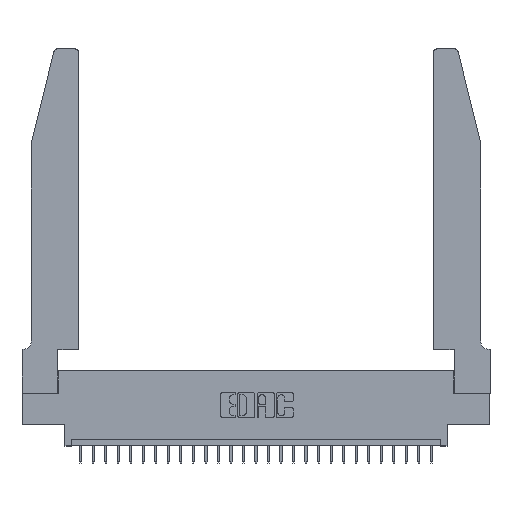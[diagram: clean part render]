
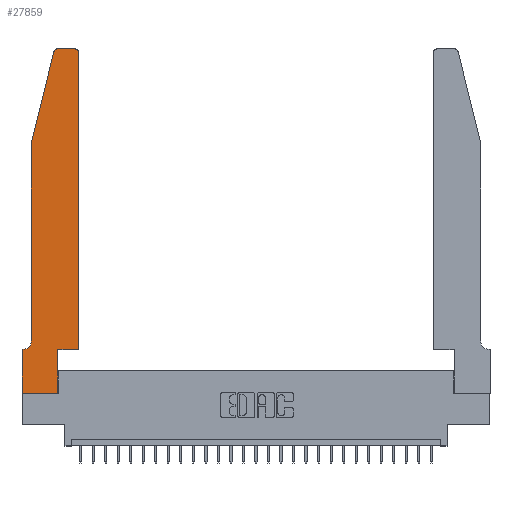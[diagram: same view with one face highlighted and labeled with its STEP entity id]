
A CAD part, top view. The second image highlights one B-rep face of the part: STEP entity #27859.
In plain terms, the highlighted planar face has unit normal (0, 0, 1).
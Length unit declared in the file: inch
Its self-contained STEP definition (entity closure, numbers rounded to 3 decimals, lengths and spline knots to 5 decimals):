
#361 = CARTESIAN_POINT ( 'NONE',  ( 0.4505, 0.35, 0.37 ) ) ;
#369 = AXIS2_PLACEMENT_3D ( 'NONE', #16245, #648, #2953 ) ;
#456 = LINE ( 'NONE', #11005, #26576 ) ;
#542 = LINE ( 'NONE', #18166, #25322 ) ;
#648 = DIRECTION ( 'NONE',  ( 0., 0., -1. ) ) ;
#783 = DIRECTION ( 'NONE',  ( 1., 0., 0. ) ) ;
#1442 = VECTOR ( 'NONE', #6772, 39.37008 ) ;
#1499 = VECTOR ( 'NONE', #19716, 39.37008 ) ;
#1533 = EDGE_CURVE ( 'NONE', #22584, #27762, #24701, .T. ) ;
#1870 = VERTEX_POINT ( 'NONE', #19478 ) ;
#1939 = PLANE ( 'NONE',  #6415 ) ;
#2054 = VERTEX_POINT ( 'NONE', #26553 ) ;
#2544 = DIRECTION ( 'NONE',  ( -0.239, -0.971, 0. ) ) ;
#2953 = DIRECTION ( 'NONE',  ( -1., 0., 0. ) ) ;
#3086 = ORIENTED_EDGE ( 'NONE', *, *, #11861, .T. ) ;
#3367 = CARTESIAN_POINT ( 'NONE',  ( 0.284, 2.72, 0.37 ) ) ;
#3793 = EDGE_CURVE ( 'NONE', #7528, #2054, #24364, .T. ) ;
#4366 = ORIENTED_EDGE ( 'NONE', *, *, #24032, .T. ) ;
#4650 = CARTESIAN_POINT ( 'NONE',  ( 0., 0., 0.37 ) ) ;
#4769 = VECTOR ( 'NONE', #24494, 39.37008 ) ;
#5351 = VECTOR ( 'NONE', #783, 39.37008 ) ;
#5953 = ORIENTED_EDGE ( 'NONE', *, *, #17704, .T. ) ;
#6149 = ORIENTED_EDGE ( 'NONE', *, *, #26749, .T. ) ;
#6403 = CARTESIAN_POINT ( 'NONE',  ( 0., 0.35, 0.37 ) ) ;
#6415 = AXIS2_PLACEMENT_3D ( 'NONE', #6403, #8720, #15228 ) ;
#6772 = DIRECTION ( 'NONE',  ( -1., 0., 0. ) ) ;
#7038 = CARTESIAN_POINT ( 'NONE',  ( 0., 0., 0.37 ) ) ;
#7094 = DIRECTION ( 'NONE',  ( 1., 0., 0. ) ) ;
#7528 = VERTEX_POINT ( 'NONE', #22080 ) ;
#7736 = VERTEX_POINT ( 'NONE', #20895 ) ;
#7796 = VERTEX_POINT ( 'NONE', #15268 ) ;
#8121 = ORIENTED_EDGE ( 'NONE', *, *, #8553, .T. ) ;
#8229 = CIRCLE ( 'NONE', #20662, 0.03 ) ;
#8553 = EDGE_CURVE ( 'NONE', #8841, #7736, #11332, .T. ) ;
#8720 = DIRECTION ( 'NONE',  ( 0., 0., 1. ) ) ;
#8841 = VERTEX_POINT ( 'NONE', #23744 ) ;
#9435 = VECTOR ( 'NONE', #7094, 39.37008 ) ;
#9494 = VECTOR ( 'NONE', #2544, 39.37008 ) ;
#9614 = LINE ( 'NONE', #13514, #9494 ) ;
#10601 = FACE_OUTER_BOUND ( 'NONE', #12995, .T. ) ;
#10947 = EDGE_CURVE ( 'NONE', #2054, #22584, #14672, .T. ) ;
#11005 = CARTESIAN_POINT ( 'NONE',  ( 0.2605, 2.75, 0.37 ) ) ;
#11064 = CARTESIAN_POINT ( 'NONE',  ( 0.0755, 2., 0.37 ) ) ;
#11247 = AXIS2_PLACEMENT_3D ( 'NONE', #15539, #28255, #28542 ) ;
#11257 = CARTESIAN_POINT ( 'NONE',  ( 0.0755, 0.35, 0.37 ) ) ;
#11332 = LINE ( 'NONE', #361, #5351 ) ;
#11582 = CARTESIAN_POINT ( 'NONE',  ( 0., 0., 0.37 ) ) ;
#11703 = CIRCLE ( 'NONE', #11247, 0.03 ) ;
#11861 = EDGE_CURVE ( 'NONE', #7736, #20098, #542, .T. ) ;
#12822 = VERTEX_POINT ( 'NONE', #11582 ) ;
#12995 = EDGE_LOOP ( 'NONE', ( #4366, #6149, #25354, #23075, #25969, #13064, #5953, #27306, #22195, #8121, #3086, #13668 ) ) ;
#13064 = ORIENTED_EDGE ( 'NONE', *, *, #1533, .T. ) ;
#13514 = CARTESIAN_POINT ( 'NONE',  ( 0.0755, 2., 0.37 ) ) ;
#13668 = ORIENTED_EDGE ( 'NONE', *, *, #19941, .T. ) ;
#13795 = CARTESIAN_POINT ( 'NONE',  ( 0.0055, 0.35, 0.37 ) ) ;
#14672 = CIRCLE ( 'NONE', #369, 0.07 ) ;
#15228 = DIRECTION ( 'NONE',  ( 1., 0., 0. ) ) ;
#15268 = CARTESIAN_POINT ( 'NONE',  ( 0.25487, 2.72718, 0.37 ) ) ;
#15539 = CARTESIAN_POINT ( 'NONE',  ( 0.4205, 2.72, 0.37 ) ) ;
#15995 = DIRECTION ( 'NONE',  ( 0., 1., 0. ) ) ;
#16245 = CARTESIAN_POINT ( 'NONE',  ( 0.0055, 0.42, 0.37 ) ) ;
#16806 = DIRECTION ( 'NONE',  ( 1., 0., 0. ) ) ;
#17084 = DIRECTION ( 'NONE',  ( 0., 0., 1. ) ) ;
#17645 = DIRECTION ( 'NONE',  ( -1., 0., 0. ) ) ;
#17704 = EDGE_CURVE ( 'NONE', #27762, #12822, #20059, .T. ) ;
#18166 = CARTESIAN_POINT ( 'NONE',  ( 0.4505, 0.35, 0.37 ) ) ;
#18259 = EDGE_CURVE ( 'NONE', #25081, #8841, #24197, .T. ) ;
#19478 = CARTESIAN_POINT ( 'NONE',  ( 0.4205, 2.75, 0.37 ) ) ;
#19561 = CARTESIAN_POINT ( 'NONE',  ( 0., 0.35, 0.37 ) ) ;
#19716 = DIRECTION ( 'NONE',  ( 0., 1., 0. ) ) ;
#19941 = EDGE_CURVE ( 'NONE', #20098, #1870, #11703, .T. ) ;
#20059 = LINE ( 'NONE', #7038, #24100 ) ;
#20098 = VERTEX_POINT ( 'NONE', #24920 ) ;
#20490 = EDGE_CURVE ( 'NONE', #12822, #25081, #26753, .T. ) ;
#20662 = AXIS2_PLACEMENT_3D ( 'NONE', #3367, #17084, #16806 ) ;
#20782 = CARTESIAN_POINT ( 'NONE',  ( 0.2865, 0., 0.37 ) ) ;
#20895 = CARTESIAN_POINT ( 'NONE',  ( 0.4505, 0.35, 0.37 ) ) ;
#21125 = VERTEX_POINT ( 'NONE', #23063 ) ;
#22080 = CARTESIAN_POINT ( 'NONE',  ( 0.0755, 2., 0.37 ) ) ;
#22195 = ORIENTED_EDGE ( 'NONE', *, *, #18259, .T. ) ;
#22584 = VERTEX_POINT ( 'NONE', #13795 ) ;
#23063 = CARTESIAN_POINT ( 'NONE',  ( 0.284, 2.75, 0.37 ) ) ;
#23075 = ORIENTED_EDGE ( 'NONE', *, *, #3793, .T. ) ;
#23744 = CARTESIAN_POINT ( 'NONE',  ( 0.2865, 0.35, 0.37 ) ) ;
#23829 = EDGE_CURVE ( 'NONE', #7796, #7528, #9614, .T. ) ;
#24032 = EDGE_CURVE ( 'NONE', #1870, #21125, #456, .T. ) ;
#24100 = VECTOR ( 'NONE', #26988, 39.37008 ) ;
#24197 = LINE ( 'NONE', #28239, #1499 ) ;
#24364 = LINE ( 'NONE', #11064, #4769 ) ;
#24494 = DIRECTION ( 'NONE',  ( 0., -1., 0. ) ) ;
#24701 = LINE ( 'NONE', #11257, #1442 ) ;
#24920 = CARTESIAN_POINT ( 'NONE',  ( 0.4505, 2.72, 0.37 ) ) ;
#25081 = VERTEX_POINT ( 'NONE', #20782 ) ;
#25322 = VECTOR ( 'NONE', #15995, 39.37008 ) ;
#25354 = ORIENTED_EDGE ( 'NONE', *, *, #23829, .T. ) ;
#25969 = ORIENTED_EDGE ( 'NONE', *, *, #10947, .T. ) ;
#26553 = CARTESIAN_POINT ( 'NONE',  ( 0.0755, 0.42, 0.37 ) ) ;
#26576 = VECTOR ( 'NONE', #17645, 39.37008 ) ;
#26749 = EDGE_CURVE ( 'NONE', #21125, #7796, #8229, .T. ) ;
#26753 = LINE ( 'NONE', #4650, #9435 ) ;
#26988 = DIRECTION ( 'NONE',  ( 0., -1., 0. ) ) ;
#27306 = ORIENTED_EDGE ( 'NONE', *, *, #20490, .T. ) ;
#27762 = VERTEX_POINT ( 'NONE', #19561 ) ;
#27859 = ADVANCED_FACE ( 'NONE', ( #10601 ), #1939, .T. ) ;
#28239 = CARTESIAN_POINT ( 'NONE',  ( 0.2865, 0.35, 0.37 ) ) ;
#28255 = DIRECTION ( 'NONE',  ( 0., 0., 1. ) ) ;
#28542 = DIRECTION ( 'NONE',  ( 1., 0., 0. ) ) ;
